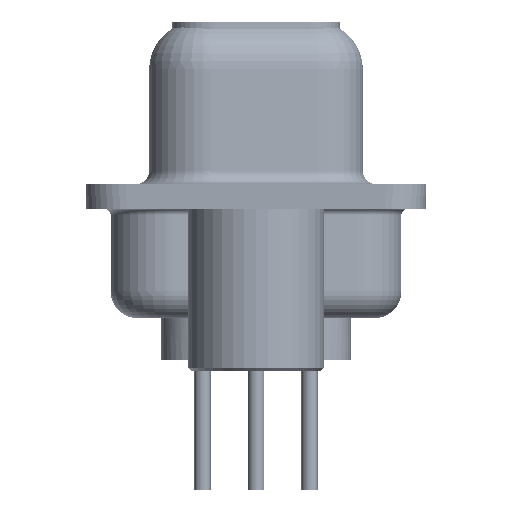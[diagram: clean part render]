
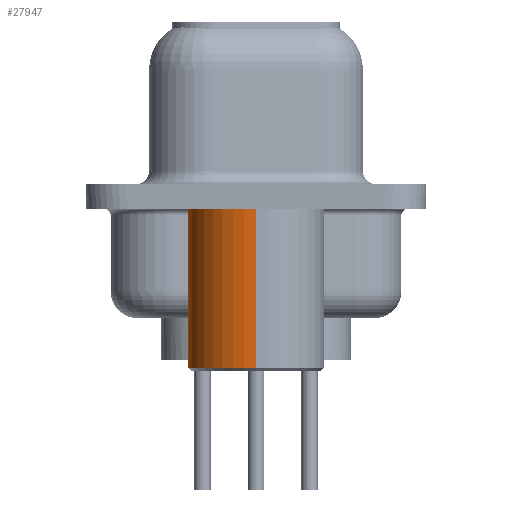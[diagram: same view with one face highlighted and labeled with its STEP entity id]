
A CAD part, left-side view. The second image highlights one B-rep face of the part: STEP entity #27947.
In plain terms, the highlighted cylindrical face has radius 2.5 mm (diameter 5 mm), a partial arc.
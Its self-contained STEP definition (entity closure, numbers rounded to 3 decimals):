
#565 = EDGE_CURVE ( 'NONE', #6140, #31982, #30344, .T. ) ;
#1195 = CARTESIAN_POINT ( 'NONE',  ( 0., 0., 0.581 ) ) ;
#2108 = CIRCLE ( 'NONE', #24817, 2.5 ) ;
#3263 = ORIENTED_EDGE ( 'NONE', *, *, #24499, .T. ) ;
#3585 = AXIS2_PLACEMENT_3D ( 'NONE', #32247, #24789, #32578 ) ;
#3801 = VECTOR ( 'NONE', #18384, 1000. ) ;
#4271 = CARTESIAN_POINT ( 'NONE',  ( -2.5, 0., -0.45 ) ) ;
#4696 = DIRECTION ( 'NONE',  ( 0., 0., 1. ) ) ;
#6140 = VERTEX_POINT ( 'NONE', #13469 ) ;
#8778 = EDGE_CURVE ( 'NONE', #31982, #11703, #2108, .T. ) ;
#9621 = DIRECTION ( 'NONE',  ( 1., 0., 0. ) ) ;
#11703 = VERTEX_POINT ( 'NONE', #4271 ) ;
#12246 = ORIENTED_EDGE ( 'NONE', *, *, #8778, .F. ) ;
#12423 = EDGE_LOOP ( 'NONE', ( #19335, #3263, #12246, #14261 ) ) ;
#13161 = CARTESIAN_POINT ( 'NONE',  ( -2.5, 0., -6.35 ) ) ;
#13462 = LINE ( 'NONE', #21253, #3801 ) ;
#13469 = CARTESIAN_POINT ( 'NONE',  ( 2.5, 0., -6.35 ) ) ;
#14261 = ORIENTED_EDGE ( 'NONE', *, *, #565, .F. ) ;
#17150 = CARTESIAN_POINT ( 'NONE',  ( 2.5, 0., 0.581 ) ) ;
#18384 = DIRECTION ( 'NONE',  ( 0., 0., 1. ) ) ;
#19335 = ORIENTED_EDGE ( 'NONE', *, *, #20464, .T. ) ;
#20464 = EDGE_CURVE ( 'NONE', #6140, #32657, #26837, .T. ) ;
#21253 = CARTESIAN_POINT ( 'NONE',  ( -2.5, 0., 0.581 ) ) ;
#24343 = CYLINDRICAL_SURFACE ( 'NONE', #30361, 2.5 ) ;
#24499 = EDGE_CURVE ( 'NONE', #32657, #11703, #13462, .T. ) ;
#24778 = DIRECTION ( 'NONE',  ( 0., 0., 1. ) ) ;
#24789 = DIRECTION ( 'NONE',  ( 0., 0., 1. ) ) ;
#24817 = AXIS2_PLACEMENT_3D ( 'NONE', #28058, #4696, #9621 ) ;
#26837 = CIRCLE ( 'NONE', #3585, 2.5 ) ;
#27943 = VECTOR ( 'NONE', #24778, 1000. ) ;
#27947 = ADVANCED_FACE ( 'NONE', ( #32144 ), #24343, .T. ) ;
#28058 = CARTESIAN_POINT ( 'NONE',  ( 0., 0., -0.45 ) ) ;
#28924 = DIRECTION ( 'NONE',  ( 0., 0., 1. ) ) ;
#29259 = DIRECTION ( 'NONE',  ( 1., 0., 0. ) ) ;
#30344 = LINE ( 'NONE', #17150, #27943 ) ;
#30361 = AXIS2_PLACEMENT_3D ( 'NONE', #1195, #28924, #29259 ) ;
#31982 = VERTEX_POINT ( 'NONE', #33264 ) ;
#32144 = FACE_OUTER_BOUND ( 'NONE', #12423, .T. ) ;
#32247 = CARTESIAN_POINT ( 'NONE',  ( 0., 0., -6.35 ) ) ;
#32578 = DIRECTION ( 'NONE',  ( 1., 0., 0. ) ) ;
#32657 = VERTEX_POINT ( 'NONE', #13161 ) ;
#33264 = CARTESIAN_POINT ( 'NONE',  ( 2.5, 0., -0.45 ) ) ;
